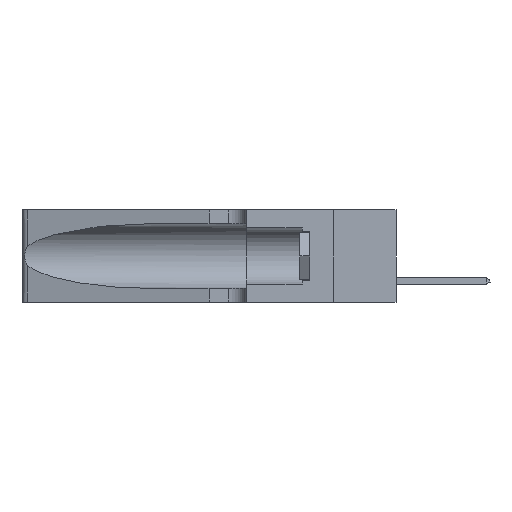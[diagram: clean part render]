
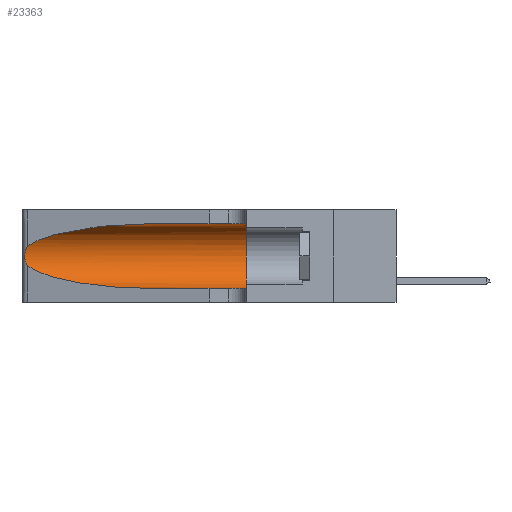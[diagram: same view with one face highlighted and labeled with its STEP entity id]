
A CAD part, left-side view. The second image highlights one B-rep face of the part: STEP entity #23363.
In plain terms, the highlighted cylindrical face has radius 3.308 mm (diameter 6.617 mm), a partial arc.
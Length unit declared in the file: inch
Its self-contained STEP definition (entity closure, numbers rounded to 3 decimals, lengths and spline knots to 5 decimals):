
#1205 = CARTESIAN_POINT ( 'NONE',  ( 0.2373, 1.15595, 0.28018 ) ) ;
#2317 = CARTESIAN_POINT ( 'NONE',  ( 0.25854, 1.2359, 0.20912 ) ) ;
#3407 = CYLINDRICAL_SURFACE ( 'NONE', #11924, 0.13025 ) ;
#3722 = ORIENTED_EDGE ( 'NONE', *, *, #13086, .F. ) ;
#4842 = VERTEX_POINT ( 'NONE', #18467 ) ;
#5030 = CARTESIAN_POINT ( 'NONE',  ( 0.25639, 1.23184, 0.21858 ) ) ;
#5256 = CARTESIAN_POINT ( 'NONE',  ( 0.1305, 0.72297, 0.05475 ) ) ;
#5536 = ORIENTED_EDGE ( 'NONE', *, *, #21628, .T. ) ;
#6431 = CARTESIAN_POINT ( 'NONE',  ( 0.1305, 0.72297, 0.05475 ) ) ;
#7985 = CIRCLE ( 'NONE', #22613, 0.13025 ) ;
#8682 = LINE ( 'NONE', #29592, #26467 ) ;
#9793 = ORIENTED_EDGE ( 'NONE', *, *, #33777, .T. ) ;
#9890 = CARTESIAN_POINT ( 'NONE',  ( 0.18966, 0.96281, 0.31525 ) ) ;
#9984 = CARTESIAN_POINT ( 'NONE',  ( 0.25487, 1.22718, 0.14631 ) ) ;
#10185 =( BOUNDED_CURVE ( )  B_SPLINE_CURVE ( 3, ( #16547, #36516, #19407, #5256 ),
 .UNSPECIFIED., .F., .T. ) 
 B_SPLINE_CURVE_WITH_KNOTS ( ( 4, 4 ),
 ( 3.44316, 4.71239 ),
 .UNSPECIFIED. ) 
 CURVE ( )  GEOMETRIC_REPRESENTATION_ITEM ( )  RATIONAL_B_SPLINE_CURVE ( ( 1., 0.87, 0.87, 1. ) ) 
 REPRESENTATION_ITEM ( '' )  );
#10657 = CARTESIAN_POINT ( 'NONE',  ( 0.25487, 1.22718, 0.22369 ) ) ;
#11256 = CARTESIAN_POINT ( 'NONE',  ( 0.26017, 1.23833, 0.17102 ) ) ;
#11924 = AXIS2_PLACEMENT_3D ( 'NONE', #32664, #24238, #27131 ) ;
#11957 = EDGE_LOOP ( 'NONE', ( #9793, #27237, #5536, #22507, #3722, #24967 ) ) ;
#13086 = EDGE_CURVE ( 'NONE', #14754, #17831, #7985, .T. ) ;
#14127 = CARTESIAN_POINT ( 'NONE',  ( 0.25555, 1.22993, 0.14849 ) ) ;
#14193 = VERTEX_POINT ( 'NONE', #6431 ) ;
#14754 = VERTEX_POINT ( 'NONE', #31182 ) ;
#14817 = EDGE_CURVE ( 'NONE', #14193, #17831, #32788, .T. ) ;
#15187 = CARTESIAN_POINT ( 'NONE',  ( 0.1305, 0.72297, 0.31525 ) ) ;
#15365 = VERTEX_POINT ( 'NONE', #9984 ) ;
#15447 = DIRECTION ( 'NONE',  ( 0., 1., 0. ) ) ;
#16465 = CARTESIAN_POINT ( 'NONE',  ( 0.25787, 1.23484, 0.2124 ) ) ;
#16547 = CARTESIAN_POINT ( 'NONE',  ( 0.25487, 1.22718, 0.14631 ) ) ;
#16935 = CARTESIAN_POINT ( 'NONE',  ( 0.25856, 1.23593, 0.16098 ) ) ;
#17831 = VERTEX_POINT ( 'NONE', #32626 ) ;
#17890 = DIRECTION ( 'NONE',  ( 0., -1., 0. ) ) ;
#18200 = CARTESIAN_POINT ( 'NONE',  ( 0.1305, 0.72297, 0.31525 ) ) ;
#18222 = DIRECTION ( 'NONE',  ( 0., -1., 0. ) ) ;
#18467 = CARTESIAN_POINT ( 'NONE',  ( 0.25487, 1.22718, 0.22369 ) ) ;
#19407 = CARTESIAN_POINT ( 'NONE',  ( 0.18966, 0.96281, 0.05475 ) ) ;
#19584 = EDGE_CURVE ( 'NONE', #4842, #15365, #36665, .T. ) ;
#19987 = VERTEX_POINT ( 'NONE', #15187 ) ;
#20163 = CARTESIAN_POINT ( 'NONE',  ( 0.25789, 1.23486, 0.15765 ) ) ;
#21042 = CARTESIAN_POINT ( 'NONE',  ( 0.25487, 1.22718, 0.22369 ) ) ;
#21628 = EDGE_CURVE ( 'NONE', #15365, #14193, #10185, .T. ) ;
#22160 = CARTESIAN_POINT ( 'NONE',  ( 0.26018, 1.23835, 0.19895 ) ) ;
#22507 = ORIENTED_EDGE ( 'NONE', *, *, #14817, .T. ) ;
#22613 = AXIS2_PLACEMENT_3D ( 'NONE', #30036, #15447, #35650 ) ;
#23363 = ADVANCED_FACE ( 'NONE', ( #36819 ), #3407, .F. ) ;
#24238 = DIRECTION ( 'NONE',  ( 0., -1., 0. ) ) ;
#24967 = ORIENTED_EDGE ( 'NONE', *, *, #27115, .F. ) ;
#25127 = VECTOR ( 'NONE', #17890, 39.37008 ) ;
#25753 = CARTESIAN_POINT ( 'NONE',  ( 0.25639, 1.23186, 0.15144 ) ) ;
#26467 = VECTOR ( 'NONE', #18222, 39.37008 ) ;
#27115 = EDGE_CURVE ( 'NONE', #19987, #14754, #8682, .T. ) ;
#27131 = DIRECTION ( 'NONE',  ( 0., 0., -1. ) ) ;
#27237 = ORIENTED_EDGE ( 'NONE', *, *, #19584, .T. ) ;
#28520 = CARTESIAN_POINT ( 'NONE',  ( 0.26075, 1.23896, 0.178 ) ) ;
#29592 = CARTESIAN_POINT ( 'NONE',  ( 0.1305, 1.61858, 0.31525 ) ) ;
#30036 = CARTESIAN_POINT ( 'NONE',  ( 0.1305, 0.35, 0.185 ) ) ;
#30046 =( BOUNDED_CURVE ( )  B_SPLINE_CURVE ( 3, ( #18200, #9890, #1205, #21042 ),
 .UNSPECIFIED., .F., .T. ) 
 B_SPLINE_CURVE_WITH_KNOTS ( ( 4, 4 ),
 ( 1.5708, 2.84003 ),
 .UNSPECIFIED. ) 
 CURVE ( )  GEOMETRIC_REPRESENTATION_ITEM ( )  RATIONAL_B_SPLINE_CURVE ( ( 1., 0.87, 0.87, 1. ) ) 
 REPRESENTATION_ITEM ( '' )  );
#30569 = CARTESIAN_POINT ( 'NONE',  ( 0.25555, 1.22994, 0.2215 ) ) ;
#31182 = CARTESIAN_POINT ( 'NONE',  ( 0.1305, 0.35, 0.31525 ) ) ;
#32626 = CARTESIAN_POINT ( 'NONE',  ( 0.1305, 0.35, 0.05475 ) ) ;
#32664 = CARTESIAN_POINT ( 'NONE',  ( 0.1305, 1.61858, 0.185 ) ) ;
#32788 = LINE ( 'NONE', #34793, #25127 ) ;
#33777 = EDGE_CURVE ( 'NONE', #19987, #4842, #30046, .T. ) ;
#34191 = CARTESIAN_POINT ( 'NONE',  ( 0.26075, 1.23896, 0.19203 ) ) ;
#34304 = CARTESIAN_POINT ( 'NONE',  ( 0.25487, 1.22718, 0.14631 ) ) ;
#34793 = CARTESIAN_POINT ( 'NONE',  ( 0.1305, 1.61858, 0.05475 ) ) ;
#35650 = DIRECTION ( 'NONE',  ( 0., 0., 1. ) ) ;
#36516 = CARTESIAN_POINT ( 'NONE',  ( 0.2373, 1.15595, 0.08982 ) ) ;
#36665 = B_SPLINE_CURVE_WITH_KNOTS ( 'NONE', 3,
 ( #10657, #30569, #5030, #16465, #2317, #22160, #34191, #28520, #11256, #16935, #20163, #25753, #14127, #34304 ),
 .UNSPECIFIED., .F., .F.,
 ( 4, 2, 2, 2, 2, 2, 4 ),
 ( 0., 0.00027, 0.00053, 0.00107, 0.0016, 0.00187, 0.00214 ),
 .UNSPECIFIED. ) ;
#36819 = FACE_OUTER_BOUND ( 'NONE', #11957, .T. ) ;
